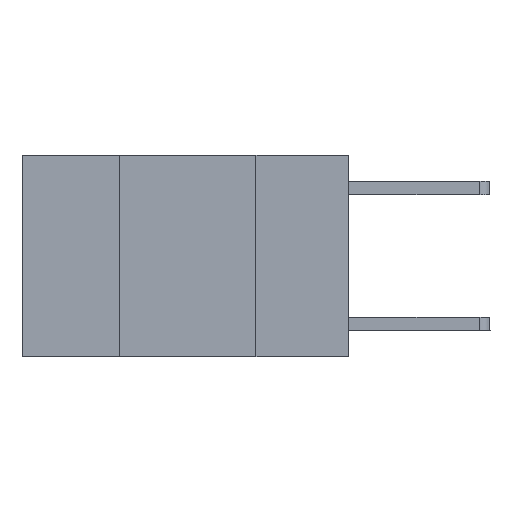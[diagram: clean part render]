
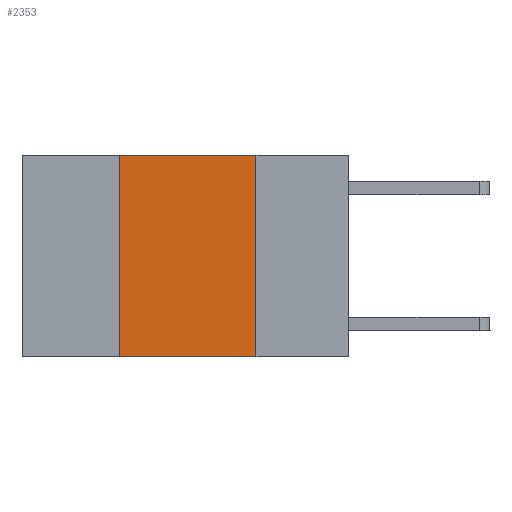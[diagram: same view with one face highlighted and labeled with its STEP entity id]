
A CAD part, left-side view. The second image highlights one B-rep face of the part: STEP entity #2353.
In plain terms, the highlighted planar face has unit normal (-1, 0, 0).
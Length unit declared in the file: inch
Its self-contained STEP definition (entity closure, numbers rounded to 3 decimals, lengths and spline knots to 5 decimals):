
#310 = CARTESIAN_POINT ( 'NONE',  ( 0., 0.6, -0.37 ) ) ;
#437 = ORIENTED_EDGE ( 'NONE', *, *, #6907, .F. ) ;
#876 = LINE ( 'NONE', #6002, #9099 ) ;
#940 = DIRECTION ( 'NONE',  ( 0., 0., -1. ) ) ;
#1098 = VECTOR ( 'NONE', #5640, 39.37008 ) ;
#1335 = VERTEX_POINT ( 'NONE', #4801 ) ;
#1466 = ORIENTED_EDGE ( 'NONE', *, *, #7475, .T. ) ;
#1618 = VECTOR ( 'NONE', #9094, 39.37008 ) ;
#1625 = VERTEX_POINT ( 'NONE', #5787 ) ;
#1820 = EDGE_LOOP ( 'NONE', ( #437, #4314, #2049, #1466 ) ) ;
#2049 = ORIENTED_EDGE ( 'NONE', *, *, #4573, .F. ) ;
#2353 = ADVANCED_FACE ( 'NONE', ( #6225 ), #9585, .F. ) ;
#3251 = VERTEX_POINT ( 'NONE', #5855 ) ;
#3578 = CARTESIAN_POINT ( 'NONE',  ( 0., 0.6, 0. ) ) ;
#3778 = CARTESIAN_POINT ( 'NONE',  ( 0., 0.6, 0. ) ) ;
#4314 = ORIENTED_EDGE ( 'NONE', *, *, #7444, .F. ) ;
#4573 = EDGE_CURVE ( 'NONE', #1335, #9030, #876, .T. ) ;
#4801 = CARTESIAN_POINT ( 'NONE',  ( 0., 0.42, -0.37 ) ) ;
#5640 = DIRECTION ( 'NONE',  ( 0., 0., -1. ) ) ;
#5787 = CARTESIAN_POINT ( 'NONE',  ( 0., 0.17, 0. ) ) ;
#5853 = DIRECTION ( 'NONE',  ( 1., 0., 0. ) ) ;
#5855 = CARTESIAN_POINT ( 'NONE',  ( 0., 0.17, -0.37 ) ) ;
#6002 = CARTESIAN_POINT ( 'NONE',  ( 0., 0.42, 0. ) ) ;
#6225 = FACE_OUTER_BOUND ( 'NONE', #1820, .T. ) ;
#6411 = CARTESIAN_POINT ( 'NONE',  ( 0., 0.17, 0. ) ) ;
#6902 = AXIS2_PLACEMENT_3D ( 'NONE', #3578, #5853, #940 ) ;
#6907 = EDGE_CURVE ( 'NONE', #1625, #3251, #9711, .T. ) ;
#7364 = CARTESIAN_POINT ( 'NONE',  ( 0., 0.42, 0. ) ) ;
#7444 = EDGE_CURVE ( 'NONE', #9030, #1625, #7799, .T. ) ;
#7475 = EDGE_CURVE ( 'NONE', #1335, #3251, #7540, .T. ) ;
#7540 = LINE ( 'NONE', #310, #9267 ) ;
#7799 = LINE ( 'NONE', #3778, #1618 ) ;
#8372 = DIRECTION ( 'NONE',  ( 0., 0., 1. ) ) ;
#8396 = DIRECTION ( 'NONE',  ( 0., -1., 0. ) ) ;
#9030 = VERTEX_POINT ( 'NONE', #7364 ) ;
#9094 = DIRECTION ( 'NONE',  ( 0., -1., 0. ) ) ;
#9099 = VECTOR ( 'NONE', #8372, 39.37008 ) ;
#9267 = VECTOR ( 'NONE', #8396, 39.37008 ) ;
#9585 = PLANE ( 'NONE',  #6902 ) ;
#9711 = LINE ( 'NONE', #6411, #1098 ) ;
